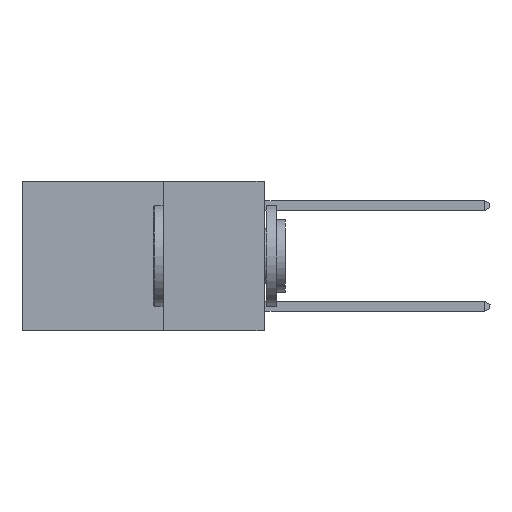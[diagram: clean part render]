
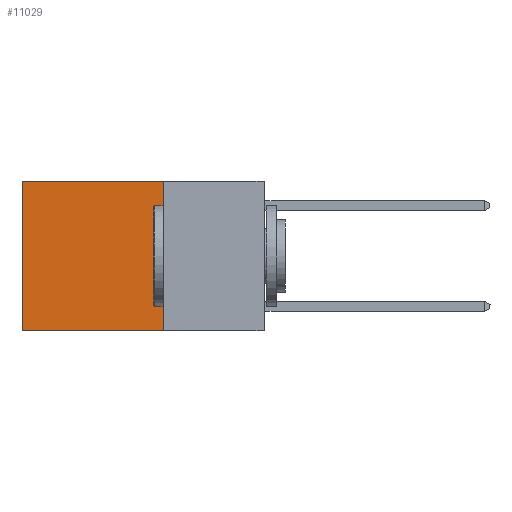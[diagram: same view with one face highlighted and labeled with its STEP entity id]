
A CAD part, left-side view. The second image highlights one B-rep face of the part: STEP entity #11029.
In plain terms, the highlighted planar face has unit normal (-1, 0, 0).
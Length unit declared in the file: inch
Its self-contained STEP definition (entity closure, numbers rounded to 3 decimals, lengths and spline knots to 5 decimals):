
#95 = EDGE_CURVE ( 'NONE', #10807, #17437, #17919, .T. ) ;
#199 = CARTESIAN_POINT ( 'NONE',  ( 0.2625, 0.25, 0. ) ) ;
#1634 = LINE ( 'NONE', #20205, #14374 ) ;
#2011 = DIRECTION ( 'NONE',  ( 0., 0., -1. ) ) ;
#2786 = LINE ( 'NONE', #21250, #19381 ) ;
#3360 = ORIENTED_EDGE ( 'NONE', *, *, #8337, .F. ) ;
#3869 = VECTOR ( 'NONE', #10445, 39.37008 ) ;
#4087 = CARTESIAN_POINT ( 'NONE',  ( 0.2625, 0.6, 0. ) ) ;
#4855 = EDGE_CURVE ( 'NONE', #13458, #18029, #1634, .T. ) ;
#7423 = CARTESIAN_POINT ( 'NONE',  ( 0.2625, 0.25, 0. ) ) ;
#8007 = CARTESIAN_POINT ( 'NONE',  ( 0.2625, 0.25, -0.37 ) ) ;
#8013 = AXIS2_PLACEMENT_3D ( 'NONE', #7423, #19024, #9102 ) ;
#8289 = LINE ( 'NONE', #18719, #3869 ) ;
#8337 = EDGE_CURVE ( 'NONE', #17437, #18029, #2786, .T. ) ;
#9102 = DIRECTION ( 'NONE',  ( 0., 0., -1. ) ) ;
#10332 = DIRECTION ( 'NONE',  ( 0., 0., -1. ) ) ;
#10445 = DIRECTION ( 'NONE',  ( 0., 1., 0. ) ) ;
#10807 = VERTEX_POINT ( 'NONE', #199 ) ;
#11029 = ADVANCED_FACE ( 'NONE', ( #18534 ), #17372, .F. ) ;
#12757 = ORIENTED_EDGE ( 'NONE', *, *, #4855, .T. ) ;
#13051 = DIRECTION ( 'NONE',  ( 0., 1., 0. ) ) ;
#13458 = VERTEX_POINT ( 'NONE', #4087 ) ;
#14374 = VECTOR ( 'NONE', #10332, 39.37008 ) ;
#14391 = ORIENTED_EDGE ( 'NONE', *, *, #14741, .T. ) ;
#14464 = EDGE_LOOP ( 'NONE', ( #12757, #3360, #20217, #14391 ) ) ;
#14741 = EDGE_CURVE ( 'NONE', #10807, #13458, #8289, .T. ) ;
#15253 = CARTESIAN_POINT ( 'NONE',  ( 0.2625, 0.25, 0. ) ) ;
#16038 = CARTESIAN_POINT ( 'NONE',  ( 0.2625, 0.6, -0.37 ) ) ;
#17372 = PLANE ( 'NONE',  #8013 ) ;
#17407 = VECTOR ( 'NONE', #2011, 39.37008 ) ;
#17437 = VERTEX_POINT ( 'NONE', #8007 ) ;
#17919 = LINE ( 'NONE', #15253, #17407 ) ;
#18029 = VERTEX_POINT ( 'NONE', #16038 ) ;
#18534 = FACE_OUTER_BOUND ( 'NONE', #14464, .T. ) ;
#18719 = CARTESIAN_POINT ( 'NONE',  ( 0.2625, 0.25, 0. ) ) ;
#19024 = DIRECTION ( 'NONE',  ( 1., 0., 0. ) ) ;
#19381 = VECTOR ( 'NONE', #13051, 39.37008 ) ;
#20205 = CARTESIAN_POINT ( 'NONE',  ( 0.2625, 0.6, 0. ) ) ;
#20217 = ORIENTED_EDGE ( 'NONE', *, *, #95, .F. ) ;
#21250 = CARTESIAN_POINT ( 'NONE',  ( 0.2625, 0.25, -0.37 ) ) ;
